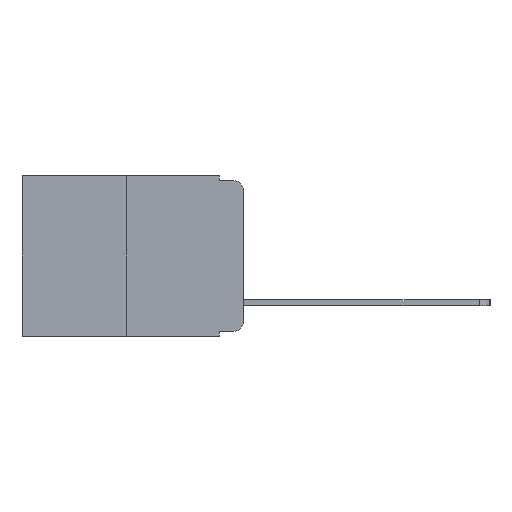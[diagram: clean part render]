
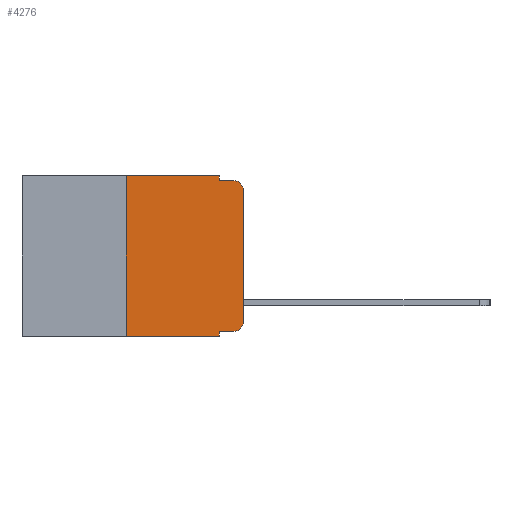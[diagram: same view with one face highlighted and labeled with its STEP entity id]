
A CAD part, left-side view. The second image highlights one B-rep face of the part: STEP entity #4276.
In plain terms, the highlighted planar face has unit normal (-1, 0, 0).
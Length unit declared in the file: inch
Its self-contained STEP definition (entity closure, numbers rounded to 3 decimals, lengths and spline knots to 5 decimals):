
#223 = CARTESIAN_POINT ( 'NONE',  ( 0., 0.051, -0.343 ) ) ;
#261 = VERTEX_POINT ( 'NONE', #5512 ) ;
#349 = CARTESIAN_POINT ( 'NONE',  ( 0., 0.473, 0. ) ) ;
#367 = DIRECTION ( 'NONE',  ( 0., 0., -1. ) ) ;
#377 = EDGE_CURVE ( 'NONE', #9039, #5945, #5315, .T. ) ;
#535 = ORIENTED_EDGE ( 'NONE', *, *, #5305, .F. ) ;
#1024 = CARTESIAN_POINT ( 'NONE',  ( 0., 0., -0.03 ) ) ;
#1078 = CARTESIAN_POINT ( 'NONE',  ( 0., 0.25, 0. ) ) ;
#1260 = ORIENTED_EDGE ( 'NONE', *, *, #9703, .T. ) ;
#1508 = VERTEX_POINT ( 'NONE', #4064 ) ;
#1569 = CARTESIAN_POINT ( 'NONE',  ( 0., 0.02, -0.313 ) ) ;
#1899 = AXIS2_PLACEMENT_3D ( 'NONE', #11181, #6001, #367 ) ;
#1994 = EDGE_CURVE ( 'NONE', #1508, #9273, #9486, .T. ) ;
#2018 = ORIENTED_EDGE ( 'NONE', *, *, #3701, .F. ) ;
#2024 = VERTEX_POINT ( 'NONE', #3136 ) ;
#2288 = VERTEX_POINT ( 'NONE', #8057 ) ;
#2338 = CARTESIAN_POINT ( 'NONE',  ( 0., 0.25, 0. ) ) ;
#2346 = VECTOR ( 'NONE', #8329, 39.37008 ) ;
#2435 = EDGE_CURVE ( 'NONE', #2024, #3967, #8005, .T. ) ;
#2517 = DIRECTION ( 'NONE',  ( 0., 0., -1. ) ) ;
#2662 = PLANE ( 'NONE',  #6534 ) ;
#2947 = ORIENTED_EDGE ( 'NONE', *, *, #377, .F. ) ;
#3009 = ORIENTED_EDGE ( 'NONE', *, *, #1994, .T. ) ;
#3024 = DIRECTION ( 'NONE',  ( 0., -1., 0. ) ) ;
#3095 = ORIENTED_EDGE ( 'NONE', *, *, #10580, .T. ) ;
#3135 = DIRECTION ( 'NONE',  ( 0., 0., -1. ) ) ;
#3136 = CARTESIAN_POINT ( 'NONE',  ( 0., 0.25, -0.343 ) ) ;
#3141 = ORIENTED_EDGE ( 'NONE', *, *, #2435, .T. ) ;
#3387 = EDGE_LOOP ( 'NONE', ( #1260, #9781, #535, #3991, #2947, #2018, #3141, #3466, #3009, #3095 ) ) ;
#3457 = VECTOR ( 'NONE', #5811, 39.37008 ) ;
#3466 = ORIENTED_EDGE ( 'NONE', *, *, #11531, .F. ) ;
#3540 = DIRECTION ( 'NONE',  ( 1., 0., 0. ) ) ;
#3579 = DIRECTION ( 'NONE',  ( 0., 0., -1. ) ) ;
#3701 = EDGE_CURVE ( 'NONE', #2024, #9039, #5879, .T. ) ;
#3967 = VERTEX_POINT ( 'NONE', #223 ) ;
#3991 = ORIENTED_EDGE ( 'NONE', *, *, #8455, .F. ) ;
#4064 = CARTESIAN_POINT ( 'NONE',  ( 0., 0.051, -0.333 ) ) ;
#4230 = CARTESIAN_POINT ( 'NONE',  ( 0., 0.051, 0. ) ) ;
#4238 = DIRECTION ( 'NONE',  ( 0., -1., 0. ) ) ;
#4276 = ADVANCED_FACE ( 'NONE', ( #5471 ), #2662, .F. ) ;
#4461 = CARTESIAN_POINT ( 'NONE',  ( 0., 0.02, -0.333 ) ) ;
#4878 = CARTESIAN_POINT ( 'NONE',  ( 0., 0.473, -0.343 ) ) ;
#4935 = CARTESIAN_POINT ( 'NONE',  ( 0., 0., -0.313 ) ) ;
#5292 = VECTOR ( 'NONE', #4238, 39.37008 ) ;
#5305 = EDGE_CURVE ( 'NONE', #2288, #261, #7955, .T. ) ;
#5315 = LINE ( 'NONE', #349, #9720 ) ;
#5471 = FACE_OUTER_BOUND ( 'NONE', #3387, .T. ) ;
#5512 = CARTESIAN_POINT ( 'NONE',  ( 0., 0.02, -0.01 ) ) ;
#5513 = LINE ( 'NONE', #4230, #7895 ) ;
#5811 = DIRECTION ( 'NONE',  ( 0., 0., 1. ) ) ;
#5879 = LINE ( 'NONE', #1078, #3457 ) ;
#5945 = VERTEX_POINT ( 'NONE', #6070 ) ;
#6001 = DIRECTION ( 'NONE',  ( -1., 0., 0. ) ) ;
#6070 = CARTESIAN_POINT ( 'NONE',  ( 0., 0.051, 0. ) ) ;
#6534 = AXIS2_PLACEMENT_3D ( 'NONE', #7202, #3540, #3579 ) ;
#6577 = VECTOR ( 'NONE', #3135, 39.37008 ) ;
#6983 = DIRECTION ( 'NONE',  ( 0., 0., -1. ) ) ;
#7198 = LINE ( 'NONE', #9196, #2346 ) ;
#7202 = CARTESIAN_POINT ( 'NONE',  ( 0., 0.473, 0. ) ) ;
#7405 = AXIS2_PLACEMENT_3D ( 'NONE', #1569, #7943, #2517 ) ;
#7588 = DIRECTION ( 'NONE',  ( 0., -1., 0. ) ) ;
#7720 = CIRCLE ( 'NONE', #7405, 0.02 ) ;
#7895 = VECTOR ( 'NONE', #6983, 39.37008 ) ;
#7943 = DIRECTION ( 'NONE',  ( -1., 0., 0. ) ) ;
#7955 = LINE ( 'NONE', #10404, #5292 ) ;
#8005 = LINE ( 'NONE', #4878, #10008 ) ;
#8057 = CARTESIAN_POINT ( 'NONE',  ( 0., 0.051, -0.01 ) ) ;
#8329 = DIRECTION ( 'NONE',  ( 0., 0., 1. ) ) ;
#8455 = EDGE_CURVE ( 'NONE', #5945, #2288, #5513, .T. ) ;
#8799 = CIRCLE ( 'NONE', #1899, 0.02 ) ;
#8829 = VERTEX_POINT ( 'NONE', #1024 ) ;
#8909 = LINE ( 'NONE', #9388, #6577 ) ;
#9039 = VERTEX_POINT ( 'NONE', #2338 ) ;
#9196 = CARTESIAN_POINT ( 'NONE',  ( 0., 0., 0. ) ) ;
#9273 = VERTEX_POINT ( 'NONE', #4461 ) ;
#9388 = CARTESIAN_POINT ( 'NONE',  ( 0., 0.051, 0. ) ) ;
#9486 = LINE ( 'NONE', #11018, #9761 ) ;
#9614 = VERTEX_POINT ( 'NONE', #4935 ) ;
#9703 = EDGE_CURVE ( 'NONE', #9614, #8829, #7198, .T. ) ;
#9720 = VECTOR ( 'NONE', #7588, 39.37008 ) ;
#9761 = VECTOR ( 'NONE', #10552, 39.37008 ) ;
#9781 = ORIENTED_EDGE ( 'NONE', *, *, #10480, .T. ) ;
#10008 = VECTOR ( 'NONE', #3024, 39.37008 ) ;
#10404 = CARTESIAN_POINT ( 'NONE',  ( 0., 0.051, -0.01 ) ) ;
#10480 = EDGE_CURVE ( 'NONE', #8829, #261, #8799, .T. ) ;
#10552 = DIRECTION ( 'NONE',  ( 0., -1., 0. ) ) ;
#10580 = EDGE_CURVE ( 'NONE', #9273, #9614, #7720, .T. ) ;
#11018 = CARTESIAN_POINT ( 'NONE',  ( 0., 0.051, -0.333 ) ) ;
#11181 = CARTESIAN_POINT ( 'NONE',  ( 0., 0.02, -0.03 ) ) ;
#11531 = EDGE_CURVE ( 'NONE', #1508, #3967, #8909, .T. ) ;
